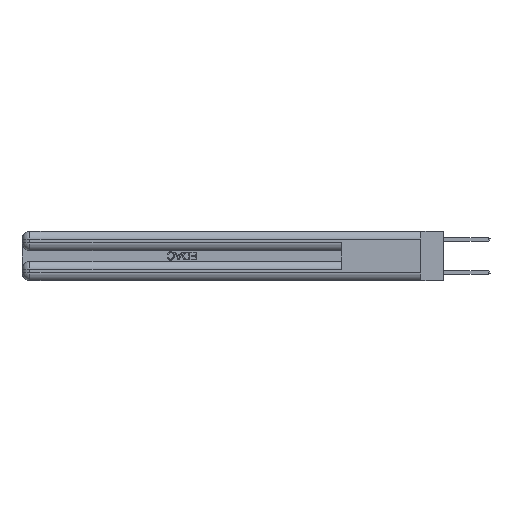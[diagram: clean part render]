
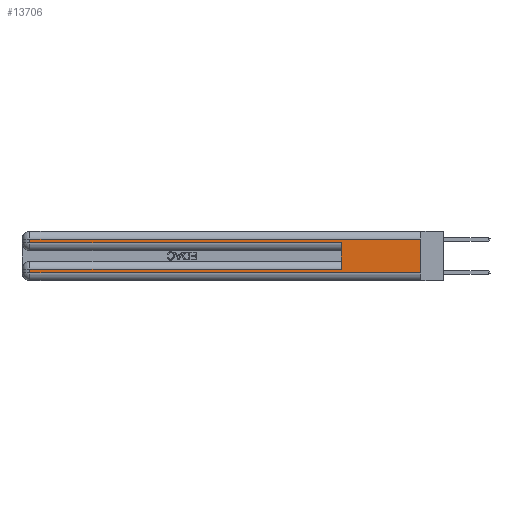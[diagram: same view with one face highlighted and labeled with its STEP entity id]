
A CAD part, left-side view. The second image highlights one B-rep face of the part: STEP entity #13706.
In plain terms, the highlighted planar face has unit normal (-1, 0, 0).
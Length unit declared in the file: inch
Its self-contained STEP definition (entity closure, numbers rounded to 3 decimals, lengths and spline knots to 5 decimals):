
#269 = VERTEX_POINT ( 'NONE', #17644 ) ;
#408 = DIRECTION ( 'NONE',  ( 0., 0., -1. ) ) ;
#597 = CARTESIAN_POINT ( 'NONE',  ( 0., 0., 0.06 ) ) ;
#1099 = CARTESIAN_POINT ( 'NONE',  ( 0., 2.94, 0.37 ) ) ;
#1283 = VERTEX_POINT ( 'NONE', #14884 ) ;
#2519 = CARTESIAN_POINT ( 'NONE',  ( 0., 2.94, 0.31 ) ) ;
#2728 = LINE ( 'NONE', #12339, #12865 ) ;
#2753 = VECTOR ( 'NONE', #13312, 39.37008 ) ;
#2944 = DIRECTION ( 'NONE',  ( 1., 0., 0. ) ) ;
#3398 = LINE ( 'NONE', #15534, #2753 ) ;
#4735 = EDGE_CURVE ( 'NONE', #5988, #269, #17679, .T. ) ;
#5159 = CARTESIAN_POINT ( 'NONE',  ( 0., 0., 0.37 ) ) ;
#5450 = VERTEX_POINT ( 'NONE', #22980 ) ;
#5967 = CARTESIAN_POINT ( 'NONE',  ( 0., 0., 0.31 ) ) ;
#5988 = VERTEX_POINT ( 'NONE', #2519 ) ;
#6540 = EDGE_CURVE ( 'NONE', #18536, #22968, #29251, .T. ) ;
#6855 = ORIENTED_EDGE ( 'NONE', *, *, #26684, .T. ) ;
#6969 = ORIENTED_EDGE ( 'NONE', *, *, #22516, .F. ) ;
#7197 = ORIENTED_EDGE ( 'NONE', *, *, #30845, .T. ) ;
#7517 = CARTESIAN_POINT ( 'NONE',  ( 0., 2.94, 0.37 ) ) ;
#7684 = ORIENTED_EDGE ( 'NONE', *, *, #4735, .T. ) ;
#8217 = DIRECTION ( 'NONE',  ( 0., 0., -1. ) ) ;
#8437 = ORIENTED_EDGE ( 'NONE', *, *, #28100, .T. ) ;
#8748 = EDGE_LOOP ( 'NONE', ( #26108, #15769, #7684, #7197, #6969, #8437, #11851, #6855 ) ) ;
#9392 = EDGE_CURVE ( 'NONE', #5450, #31041, #2728, .T. ) ;
#9894 = PLANE ( 'NONE',  #14794 ) ;
#10390 = LINE ( 'NONE', #5967, #27143 ) ;
#11851 = ORIENTED_EDGE ( 'NONE', *, *, #6540, .T. ) ;
#12235 = LINE ( 'NONE', #21885, #28603 ) ;
#12339 = CARTESIAN_POINT ( 'NONE',  ( 0., 0., 0.37 ) ) ;
#12704 = DIRECTION ( 'NONE',  ( 0., 0., 1. ) ) ;
#12865 = VECTOR ( 'NONE', #24950, 39.37008 ) ;
#13312 = DIRECTION ( 'NONE',  ( 0., 1., 0. ) ) ;
#13410 = CARTESIAN_POINT ( 'NONE',  ( 0., 0., 0.285 ) ) ;
#13706 = ADVANCED_FACE ( 'NONE', ( #16823 ), #9894, .F. ) ;
#13722 = DIRECTION ( 'NONE',  ( 0., -1., 0. ) ) ;
#14733 = LINE ( 'NONE', #17426, #20422 ) ;
#14794 = AXIS2_PLACEMENT_3D ( 'NONE', #5159, #2944, #19055 ) ;
#14884 = CARTESIAN_POINT ( 'NONE',  ( 0., 0.6, 0.285 ) ) ;
#14957 = VECTOR ( 'NONE', #13722, 39.37008 ) ;
#15534 = CARTESIAN_POINT ( 'NONE',  ( 0., 0., 0.085 ) ) ;
#15769 = ORIENTED_EDGE ( 'NONE', *, *, #23393, .T. ) ;
#16823 = FACE_OUTER_BOUND ( 'NONE', #8748, .T. ) ;
#17426 = CARTESIAN_POINT ( 'NONE',  ( 0., 0., 0.06 ) ) ;
#17565 = VERTEX_POINT ( 'NONE', #28698 ) ;
#17644 = CARTESIAN_POINT ( 'NONE',  ( 0., 2.94, 0.285 ) ) ;
#17679 = LINE ( 'NONE', #1099, #26712 ) ;
#18536 = VERTEX_POINT ( 'NONE', #29295 ) ;
#18881 = VECTOR ( 'NONE', #408, 39.37008 ) ;
#19055 = DIRECTION ( 'NONE',  ( 0., 0., -1. ) ) ;
#20422 = VECTOR ( 'NONE', #26866, 39.37008 ) ;
#21885 = CARTESIAN_POINT ( 'NONE',  ( 0., 0.6, 0.145 ) ) ;
#22516 = EDGE_CURVE ( 'NONE', #17565, #1283, #12235, .T. ) ;
#22968 = VERTEX_POINT ( 'NONE', #23521 ) ;
#22980 = CARTESIAN_POINT ( 'NONE',  ( 0., 0., 0.31 ) ) ;
#23393 = EDGE_CURVE ( 'NONE', #5450, #5988, #10390, .T. ) ;
#23521 = CARTESIAN_POINT ( 'NONE',  ( 0., 2.94, 0.06 ) ) ;
#24950 = DIRECTION ( 'NONE',  ( 0., 0., -1. ) ) ;
#26108 = ORIENTED_EDGE ( 'NONE', *, *, #9392, .F. ) ;
#26684 = EDGE_CURVE ( 'NONE', #22968, #31041, #14733, .T. ) ;
#26712 = VECTOR ( 'NONE', #8217, 39.37008 ) ;
#26866 = DIRECTION ( 'NONE',  ( 0., -1., 0. ) ) ;
#27143 = VECTOR ( 'NONE', #29610, 39.37008 ) ;
#27608 = LINE ( 'NONE', #13410, #14957 ) ;
#28100 = EDGE_CURVE ( 'NONE', #17565, #18536, #3398, .T. ) ;
#28603 = VECTOR ( 'NONE', #12704, 39.37008 ) ;
#28698 = CARTESIAN_POINT ( 'NONE',  ( 0., 0.6, 0.085 ) ) ;
#29251 = LINE ( 'NONE', #7517, #18881 ) ;
#29295 = CARTESIAN_POINT ( 'NONE',  ( 0., 2.94, 0.085 ) ) ;
#29610 = DIRECTION ( 'NONE',  ( 0., 1., 0. ) ) ;
#30845 = EDGE_CURVE ( 'NONE', #269, #1283, #27608, .T. ) ;
#31041 = VERTEX_POINT ( 'NONE', #597 ) ;
